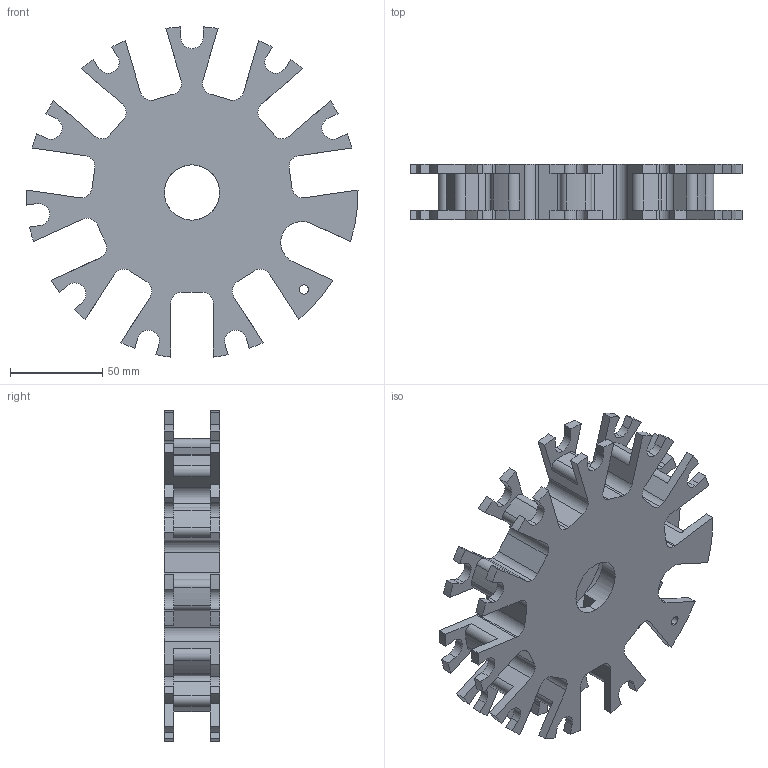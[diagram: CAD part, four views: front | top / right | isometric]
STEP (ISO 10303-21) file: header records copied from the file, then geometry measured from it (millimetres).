
FILE_DESCRIPTION (( 'STEP AP203' ), '1' );
FILE_NAME ('spindle.STEP', '2013-09-09T02:47:31', ( '' ), ( '' ), 'SwSTEP 2.0', 'SolidWorks 2013', '' );
FILE_SCHEMA (( 'CONFIG_CONTROL_DESIGN' ));
Length unit declared in the file: millimetre
Products named in the file (1): spindle
Bounding box: 179.98 x 30 x 179.06 mm (x, y, z)
Volume: 348201.5 mm3; surface area: 74240.8 mm2
Topology: 1 solids, 1 shells, 256 faces, 747 edges, 493 vertices
Faces by surface type: cylinder 145, plane 107, bspline 4
Entity records: 8877 total; most frequent: CARTESIAN_POINT 1753, DIRECTION 1542, ORIENTED_EDGE 1494, EDGE_CURVE 747, AXIS2_PLACEMENT_3D 549, VERTEX_POINT 493, LINE 444, VECTOR 444
